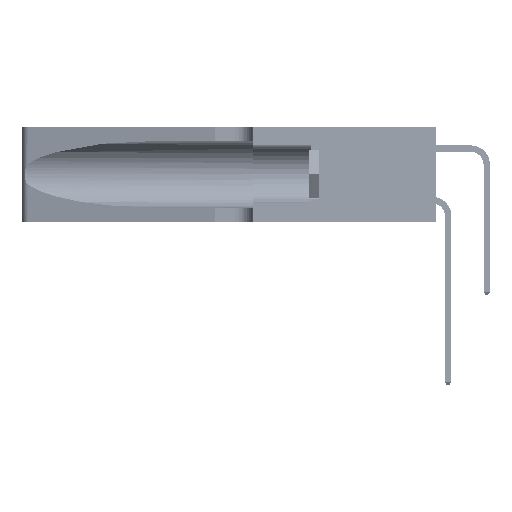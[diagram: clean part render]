
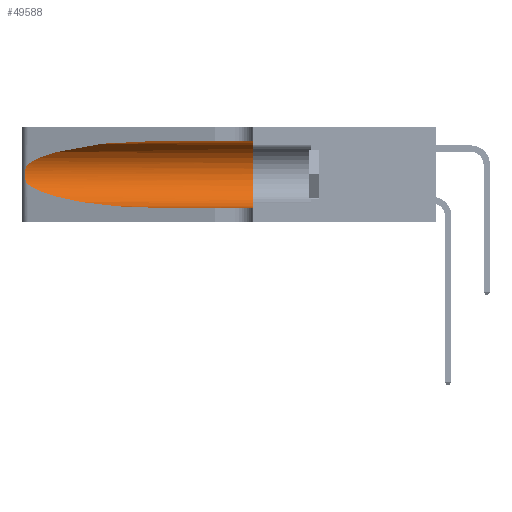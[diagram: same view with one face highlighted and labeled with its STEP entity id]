
A CAD part, left-side view. The second image highlights one B-rep face of the part: STEP entity #49588.
In plain terms, the highlighted cylindrical face has radius 3.308 mm (diameter 6.617 mm), a partial arc.
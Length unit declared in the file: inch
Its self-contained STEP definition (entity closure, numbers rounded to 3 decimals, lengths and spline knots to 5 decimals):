
#682 = ORIENTED_EDGE ( 'NONE', *, *, #42545, .T. ) ;
#754 = VERTEX_POINT ( 'NONE', #51053 ) ;
#1891 = AXIS2_PLACEMENT_3D ( 'NONE', #41660, #8676, #25573 ) ;
#2174 = CARTESIAN_POINT ( 'NONE',  ( 0.25487, 1.22718, 0.14631 ) ) ;
#2538 = CARTESIAN_POINT ( 'NONE',  ( 0.25789, 1.23486, 0.15765 ) ) ;
#2810 = AXIS2_PLACEMENT_3D ( 'NONE', #47756, #14412, #47396 ) ;
#4625 = EDGE_CURVE ( 'NONE', #16829, #47737, #32112, .T. ) ;
#6321 = CARTESIAN_POINT ( 'NONE',  ( 0.25856, 1.23593, 0.16098 ) ) ;
#6400 = ORIENTED_EDGE ( 'NONE', *, *, #18844, .T. ) ;
#6652 = CARTESIAN_POINT ( 'NONE',  ( 0.26075, 1.23896, 0.19203 ) ) ;
#7111 = CARTESIAN_POINT ( 'NONE',  ( 0.18966, 0.96281, 0.31525 ) ) ;
#7519 = LINE ( 'NONE', #37708, #49880 ) ;
#8676 = DIRECTION ( 'NONE',  ( 0., -1., 0. ) ) ;
#8999 = CIRCLE ( 'NONE', #2810, 0.13025 ) ;
#9385 = CARTESIAN_POINT ( 'NONE',  ( 0.25487, 1.22718, 0.14631 ) ) ;
#9539 = EDGE_LOOP ( 'NONE', ( #43240, #38397, #6400, #682, #10152, #25049 ) ) ;
#10152 = ORIENTED_EDGE ( 'NONE', *, *, #28667, .F. ) ;
#12306 = FACE_OUTER_BOUND ( 'NONE', #9539, .T. ) ;
#13419 = CARTESIAN_POINT ( 'NONE',  ( 0.25487, 1.22718, 0.22369 ) ) ;
#14412 = DIRECTION ( 'NONE',  ( 0., 1., 0. ) ) ;
#15538 = CARTESIAN_POINT ( 'NONE',  ( 0.1305, 0.72297, 0.31525 ) ) ;
#16829 = VERTEX_POINT ( 'NONE', #13419 ) ;
#17846 = CARTESIAN_POINT ( 'NONE',  ( 0.18966, 0.96281, 0.05475 ) ) ;
#18033 = CARTESIAN_POINT ( 'NONE',  ( 0.1305, 0.72297, 0.05475 ) ) ;
#18625 =( BOUNDED_CURVE ( )  B_SPLINE_CURVE ( 3, ( #15538, #7111, #31864, #39737 ),
 .UNSPECIFIED., .F., .F. ) 
 B_SPLINE_CURVE_WITH_KNOTS ( ( 4, 4 ),
 ( 1.5708, 2.84003 ),
 .UNSPECIFIED. ) 
 CURVE ( )  GEOMETRIC_REPRESENTATION_ITEM ( )  RATIONAL_B_SPLINE_CURVE ( ( 1., 0.87, 0.87, 1. ) ) 
 REPRESENTATION_ITEM ( '' )  );
#18844 = EDGE_CURVE ( 'NONE', #47737, #52989, #37678, .T. ) ;
#18868 = CARTESIAN_POINT ( 'NONE',  ( 0.25555, 1.22994, 0.2215 ) ) ;
#19930 = CARTESIAN_POINT ( 'NONE',  ( 0.1305, 0.35, 0.31525 ) ) ;
#22818 = CARTESIAN_POINT ( 'NONE',  ( 0.25854, 1.2359, 0.20912 ) ) ;
#23341 = CARTESIAN_POINT ( 'NONE',  ( 0.26017, 1.23833, 0.17102 ) ) ;
#24065 = VECTOR ( 'NONE', #40964, 39.37008 ) ;
#25049 = ORIENTED_EDGE ( 'NONE', *, *, #41414, .F. ) ;
#25573 = DIRECTION ( 'NONE',  ( 0., 0., -1. ) ) ;
#27481 = CARTESIAN_POINT ( 'NONE',  ( 0.25639, 1.23186, 0.15144 ) ) ;
#28667 = EDGE_CURVE ( 'NONE', #45574, #50336, #8999, .T. ) ;
#29025 = CARTESIAN_POINT ( 'NONE',  ( 0.1305, 0.35, 0.05475 ) ) ;
#29649 = DIRECTION ( 'NONE',  ( 0., -1., 0. ) ) ;
#30059 = CARTESIAN_POINT ( 'NONE',  ( 0.25487, 1.22718, 0.14631 ) ) ;
#30878 = CARTESIAN_POINT ( 'NONE',  ( 0.25555, 1.22993, 0.14849 ) ) ;
#31864 = CARTESIAN_POINT ( 'NONE',  ( 0.2373, 1.15595, 0.28018 ) ) ;
#32112 = B_SPLINE_CURVE_WITH_KNOTS ( 'NONE', 3,
 ( #34800, #18868, #43233, #47369, #22818, #39285, #6652, #43604, #23341, #6321, #2538, #27481, #30878, #2174 ),
 .UNSPECIFIED., .F., .F.,
 ( 4, 2, 2, 2, 2, 2, 4 ),
 ( 0., 0.00027, 0.00053, 0.00107, 0.0016, 0.00187, 0.00214 ),
 .UNSPECIFIED. ) ;
#34800 = CARTESIAN_POINT ( 'NONE',  ( 0.25487, 1.22718, 0.22369 ) ) ;
#36290 = LINE ( 'NONE', #36868, #24065 ) ;
#36868 = CARTESIAN_POINT ( 'NONE',  ( 0.1305, 1.61858, 0.05475 ) ) ;
#37678 =( BOUNDED_CURVE ( )  B_SPLINE_CURVE ( 3, ( #9385, #50129, #17846, #18033 ),
 .UNSPECIFIED., .F., .F. ) 
 B_SPLINE_CURVE_WITH_KNOTS ( ( 4, 4 ),
 ( 3.44316, 4.71239 ),
 .UNSPECIFIED. ) 
 CURVE ( )  GEOMETRIC_REPRESENTATION_ITEM ( )  RATIONAL_B_SPLINE_CURVE ( ( 1., 0.87, 0.87, 1. ) ) 
 REPRESENTATION_ITEM ( '' )  );
#37708 = CARTESIAN_POINT ( 'NONE',  ( 0.1305, 1.61858, 0.31525 ) ) ;
#37709 = EDGE_CURVE ( 'NONE', #754, #16829, #18625, .T. ) ;
#38397 = ORIENTED_EDGE ( 'NONE', *, *, #4625, .T. ) ;
#39285 = CARTESIAN_POINT ( 'NONE',  ( 0.26018, 1.23835, 0.19895 ) ) ;
#39737 = CARTESIAN_POINT ( 'NONE',  ( 0.25487, 1.22718, 0.22369 ) ) ;
#40964 = DIRECTION ( 'NONE',  ( 0., -1., 0. ) ) ;
#41414 = EDGE_CURVE ( 'NONE', #754, #45574, #7519, .T. ) ;
#41660 = CARTESIAN_POINT ( 'NONE',  ( 0.1305, 1.61858, 0.185 ) ) ;
#42545 = EDGE_CURVE ( 'NONE', #52989, #50336, #36290, .T. ) ;
#43233 = CARTESIAN_POINT ( 'NONE',  ( 0.25639, 1.23184, 0.21858 ) ) ;
#43240 = ORIENTED_EDGE ( 'NONE', *, *, #37709, .T. ) ;
#43604 = CARTESIAN_POINT ( 'NONE',  ( 0.26075, 1.23896, 0.178 ) ) ;
#45574 = VERTEX_POINT ( 'NONE', #19930 ) ;
#47369 = CARTESIAN_POINT ( 'NONE',  ( 0.25787, 1.23484, 0.2124 ) ) ;
#47396 = DIRECTION ( 'NONE',  ( 0., 0., 1. ) ) ;
#47737 = VERTEX_POINT ( 'NONE', #30059 ) ;
#47756 = CARTESIAN_POINT ( 'NONE',  ( 0.1305, 0.35, 0.185 ) ) ;
#49578 = CARTESIAN_POINT ( 'NONE',  ( 0.1305, 0.72297, 0.05475 ) ) ;
#49588 = ADVANCED_FACE ( 'NONE', ( #12306 ), #50825, .F. ) ;
#49880 = VECTOR ( 'NONE', #29649, 39.37008 ) ;
#50129 = CARTESIAN_POINT ( 'NONE',  ( 0.2373, 1.15595, 0.08982 ) ) ;
#50336 = VERTEX_POINT ( 'NONE', #29025 ) ;
#50825 = CYLINDRICAL_SURFACE ( 'NONE', #1891, 0.13025 ) ;
#51053 = CARTESIAN_POINT ( 'NONE',  ( 0.1305, 0.72297, 0.31525 ) ) ;
#52989 = VERTEX_POINT ( 'NONE', #49578 ) ;
